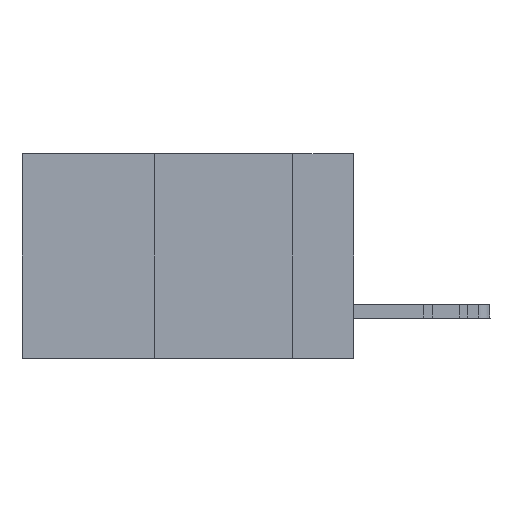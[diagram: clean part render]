
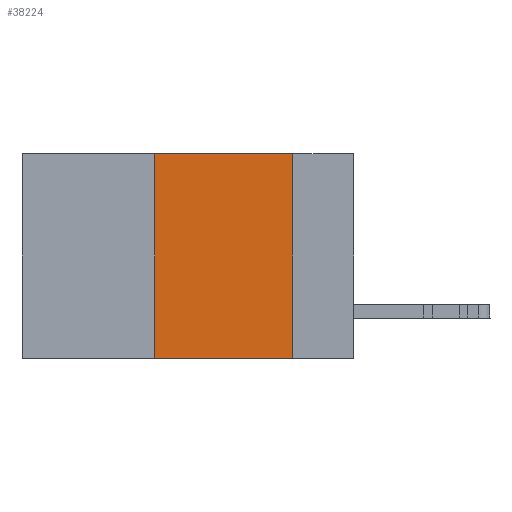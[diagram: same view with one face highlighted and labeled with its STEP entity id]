
A CAD part, left-side view. The second image highlights one B-rep face of the part: STEP entity #38224.
In plain terms, the highlighted planar face has unit normal (-1, 0, 0).
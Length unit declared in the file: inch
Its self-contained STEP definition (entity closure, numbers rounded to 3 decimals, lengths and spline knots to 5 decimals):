
#1779 = DIRECTION ( 'NONE',  ( 0., 0., -1. ) ) ;
#2057 = PLANE ( 'NONE',  #11706 ) ;
#2251 = EDGE_CURVE ( 'NONE', #21281, #9530, #38864, .T. ) ;
#3334 = DIRECTION ( 'NONE',  ( 0., -1., 0. ) ) ;
#3379 = CARTESIAN_POINT ( 'NONE',  ( 0., 0.36, 0. ) ) ;
#3472 = ORIENTED_EDGE ( 'NONE', *, *, #36719, .T. ) ;
#3478 = CARTESIAN_POINT ( 'NONE',  ( 0., 0.6, -0.37 ) ) ;
#4151 = VECTOR ( 'NONE', #8018, 39.37008 ) ;
#6325 = LINE ( 'NONE', #21876, #4151 ) ;
#6596 = EDGE_CURVE ( 'NONE', #41310, #21281, #6325, .T. ) ;
#8018 = DIRECTION ( 'NONE',  ( 0., -1., 0. ) ) ;
#9530 = VERTEX_POINT ( 'NONE', #25202 ) ;
#9895 = ORIENTED_EDGE ( 'NONE', *, *, #2251, .F. ) ;
#11706 = AXIS2_PLACEMENT_3D ( 'NONE', #35971, #12165, #1779 ) ;
#12165 = DIRECTION ( 'NONE',  ( 1., 0., 0. ) ) ;
#12567 = VECTOR ( 'NONE', #37568, 39.37008 ) ;
#14049 = LINE ( 'NONE', #3478, #40450 ) ;
#18053 = EDGE_CURVE ( 'NONE', #27655, #41310, #25495, .T. ) ;
#20091 = CARTESIAN_POINT ( 'NONE',  ( 0., 0.36, 0. ) ) ;
#21281 = VERTEX_POINT ( 'NONE', #34029 ) ;
#21876 = CARTESIAN_POINT ( 'NONE',  ( 0., 0.6, 0. ) ) ;
#24230 = ORIENTED_EDGE ( 'NONE', *, *, #18053, .F. ) ;
#25202 = CARTESIAN_POINT ( 'NONE',  ( 0., 0.11, -0.37 ) ) ;
#25495 = LINE ( 'NONE', #20091, #12567 ) ;
#27655 = VERTEX_POINT ( 'NONE', #39139 ) ;
#29296 = EDGE_LOOP ( 'NONE', ( #9895, #37941, #24230, #3472 ) ) ;
#34029 = CARTESIAN_POINT ( 'NONE',  ( 0., 0.11, 0. ) ) ;
#35236 = CARTESIAN_POINT ( 'NONE',  ( 0., 0.11, 0. ) ) ;
#35971 = CARTESIAN_POINT ( 'NONE',  ( 0., 0.6, 0. ) ) ;
#36719 = EDGE_CURVE ( 'NONE', #27655, #9530, #14049, .T. ) ;
#37568 = DIRECTION ( 'NONE',  ( 0., 0., 1. ) ) ;
#37785 = VECTOR ( 'NONE', #38699, 39.37008 ) ;
#37941 = ORIENTED_EDGE ( 'NONE', *, *, #6596, .F. ) ;
#38123 = FACE_OUTER_BOUND ( 'NONE', #29296, .T. ) ;
#38224 = ADVANCED_FACE ( 'NONE', ( #38123 ), #2057, .F. ) ;
#38699 = DIRECTION ( 'NONE',  ( 0., 0., -1. ) ) ;
#38864 = LINE ( 'NONE', #35236, #37785 ) ;
#39139 = CARTESIAN_POINT ( 'NONE',  ( 0., 0.36, -0.37 ) ) ;
#40450 = VECTOR ( 'NONE', #3334, 39.37008 ) ;
#41310 = VERTEX_POINT ( 'NONE', #3379 ) ;
